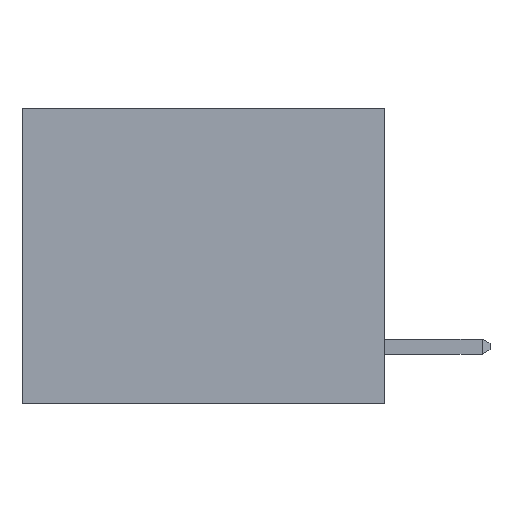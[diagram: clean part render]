
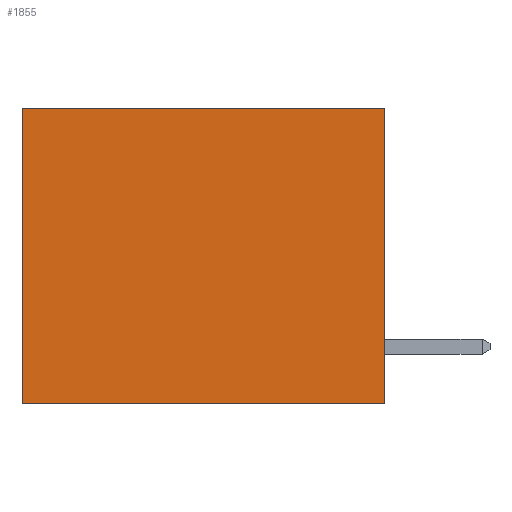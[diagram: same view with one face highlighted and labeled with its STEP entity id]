
A CAD part, left-side view. The second image highlights one B-rep face of the part: STEP entity #1855.
In plain terms, the highlighted planar face has unit normal (-1, 0, 0).
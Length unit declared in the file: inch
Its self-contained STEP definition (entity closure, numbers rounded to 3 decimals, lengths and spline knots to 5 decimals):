
#218 = VERTEX_POINT ( 'NONE', #1707 ) ;
#277 = ORIENTED_EDGE ( 'NONE', *, *, #2100, .T. ) ;
#372 = DIRECTION ( 'NONE',  ( 1., 0., 0. ) ) ;
#796 = PLANE ( 'NONE',  #1731 ) ;
#1358 = VECTOR ( 'NONE', #5660, 39.37008 ) ;
#1707 = CARTESIAN_POINT ( 'NONE',  ( 0.3165, 0., -0.49 ) ) ;
#1728 = FACE_OUTER_BOUND ( 'NONE', #2932, .T. ) ;
#1731 = AXIS2_PLACEMENT_3D ( 'NONE', #3749, #372, #9701 ) ;
#1855 = ADVANCED_FACE ( 'NONE', ( #1728 ), #796, .F. ) ;
#2100 = EDGE_CURVE ( 'NONE', #7667, #7435, #8354, .T. ) ;
#2599 = ORIENTED_EDGE ( 'NONE', *, *, #2884, .T. ) ;
#2884 = EDGE_CURVE ( 'NONE', #7435, #5914, #7106, .T. ) ;
#2932 = EDGE_LOOP ( 'NONE', ( #2599, #5562, #4485, #277 ) ) ;
#3135 = CARTESIAN_POINT ( 'NONE',  ( 0.3165, 0., 0. ) ) ;
#3436 = LINE ( 'NONE', #4322, #10216 ) ;
#3749 = CARTESIAN_POINT ( 'NONE',  ( 0.3165, 0., -0.49 ) ) ;
#3779 = DIRECTION ( 'NONE',  ( 0., 0., -1. ) ) ;
#3992 = LINE ( 'NONE', #7490, #5874 ) ;
#4159 = EDGE_CURVE ( 'NONE', #218, #5914, #3992, .T. ) ;
#4322 = CARTESIAN_POINT ( 'NONE',  ( 0.3165, 0., -0.49 ) ) ;
#4485 = ORIENTED_EDGE ( 'NONE', *, *, #4808, .F. ) ;
#4808 = EDGE_CURVE ( 'NONE', #7667, #218, #3436, .T. ) ;
#5562 = ORIENTED_EDGE ( 'NONE', *, *, #4159, .F. ) ;
#5660 = DIRECTION ( 'NONE',  ( 0., 1., 0. ) ) ;
#5874 = VECTOR ( 'NONE', #10258, 39.37008 ) ;
#5914 = VERTEX_POINT ( 'NONE', #7573 ) ;
#6254 = CARTESIAN_POINT ( 'NONE',  ( 0.3165, 0.6, 0. ) ) ;
#6757 = CARTESIAN_POINT ( 'NONE',  ( 0.3165, 0.6, -0.49 ) ) ;
#7106 = LINE ( 'NONE', #6757, #7746 ) ;
#7435 = VERTEX_POINT ( 'NONE', #6254 ) ;
#7490 = CARTESIAN_POINT ( 'NONE',  ( 0.3165, 0., -0.49 ) ) ;
#7573 = CARTESIAN_POINT ( 'NONE',  ( 0.3165, 0.6, -0.49 ) ) ;
#7667 = VERTEX_POINT ( 'NONE', #3135 ) ;
#7746 = VECTOR ( 'NONE', #8396, 39.37008 ) ;
#8354 = LINE ( 'NONE', #9001, #1358 ) ;
#8396 = DIRECTION ( 'NONE',  ( 0., 0., -1. ) ) ;
#9001 = CARTESIAN_POINT ( 'NONE',  ( 0.3165, 0., 0. ) ) ;
#9701 = DIRECTION ( 'NONE',  ( 0., 0., -1. ) ) ;
#10216 = VECTOR ( 'NONE', #3779, 39.37008 ) ;
#10258 = DIRECTION ( 'NONE',  ( 0., 1., 0. ) ) ;
